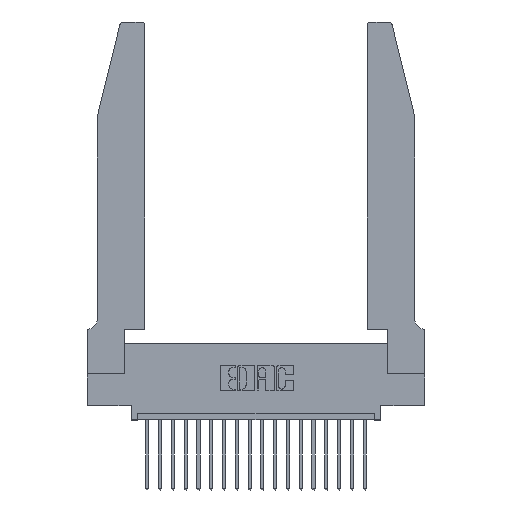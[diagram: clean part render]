
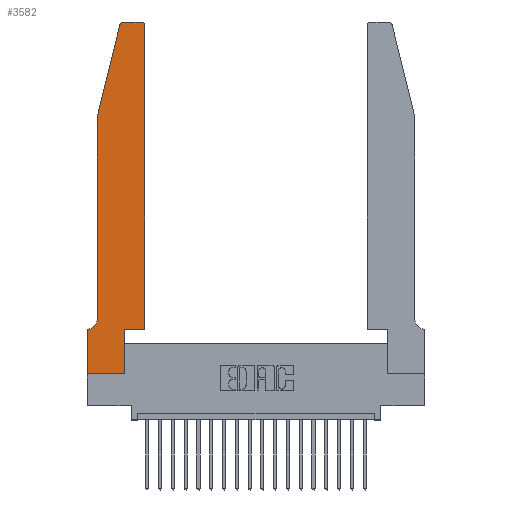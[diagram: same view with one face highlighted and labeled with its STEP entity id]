
A CAD part, top view. The second image highlights one B-rep face of the part: STEP entity #3582.
In plain terms, the highlighted planar face has unit normal (0, 0, 1).
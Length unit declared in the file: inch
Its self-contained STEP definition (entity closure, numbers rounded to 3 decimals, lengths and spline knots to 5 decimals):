
#22 = AXIS2_PLACEMENT_3D ( 'NONE', #5858, #7296, #2574 ) ;
#95 = CARTESIAN_POINT ( 'NONE',  ( 0.0755, 0.35, 0.37 ) ) ;
#312 = VERTEX_POINT ( 'NONE', #9934 ) ;
#774 = ORIENTED_EDGE ( 'NONE', *, *, #19800, .T. ) ;
#833 = ORIENTED_EDGE ( 'NONE', *, *, #8373, .T. ) ;
#1191 = CARTESIAN_POINT ( 'NONE',  ( 0.2865, 0., 0.37 ) ) ;
#1224 = DIRECTION ( 'NONE',  ( 0., 0., -1. ) ) ;
#1525 = VERTEX_POINT ( 'NONE', #7065 ) ;
#2114 = VERTEX_POINT ( 'NONE', #6592 ) ;
#2199 = DIRECTION ( 'NONE',  ( 1., 0., 0. ) ) ;
#2287 = CARTESIAN_POINT ( 'NONE',  ( 0.4505, 2.72, 0.37 ) ) ;
#2424 = CARTESIAN_POINT ( 'NONE',  ( 0.4505, 0.35, 0.37 ) ) ;
#2574 = DIRECTION ( 'NONE',  ( 1., 0., 0. ) ) ;
#2687 = CARTESIAN_POINT ( 'NONE',  ( 0., 0., 0.37 ) ) ;
#2689 = CARTESIAN_POINT ( 'NONE',  ( 0.4505, 0.35, 0.37 ) ) ;
#2951 = ORIENTED_EDGE ( 'NONE', *, *, #8413, .T. ) ;
#3290 = EDGE_CURVE ( 'NONE', #312, #1525, #5204, .T. ) ;
#3326 = CARTESIAN_POINT ( 'NONE',  ( 0.0755, 2., 0.37 ) ) ;
#3443 = DIRECTION ( 'NONE',  ( 0., 1., 0. ) ) ;
#3567 = VERTEX_POINT ( 'NONE', #18873 ) ;
#3582 = ADVANCED_FACE ( 'NONE', ( #17757 ), #12423, .T. ) ;
#4281 = CIRCLE ( 'NONE', #22, 0.03 ) ;
#4455 = EDGE_CURVE ( 'NONE', #10962, #15552, #10464, .T. ) ;
#4823 = VERTEX_POINT ( 'NONE', #2689 ) ;
#4848 = CIRCLE ( 'NONE', #10200, 0.07 ) ;
#5204 = LINE ( 'NONE', #95, #15141 ) ;
#5340 = DIRECTION ( 'NONE',  ( 1., 0., 0. ) ) ;
#5797 = ORIENTED_EDGE ( 'NONE', *, *, #17978, .T. ) ;
#5858 = CARTESIAN_POINT ( 'NONE',  ( 0.4205, 2.72, 0.37 ) ) ;
#5996 = VECTOR ( 'NONE', #9493, 39.37008 ) ;
#6002 = VERTEX_POINT ( 'NONE', #9565 ) ;
#6037 = VECTOR ( 'NONE', #3443, 39.37008 ) ;
#6434 = EDGE_CURVE ( 'NONE', #2114, #17561, #7002, .T. ) ;
#6592 = CARTESIAN_POINT ( 'NONE',  ( 0.25487, 2.72718, 0.37 ) ) ;
#6867 = DIRECTION ( 'NONE',  ( 1., 0., 0. ) ) ;
#7002 = LINE ( 'NONE', #3326, #19838 ) ;
#7065 = CARTESIAN_POINT ( 'NONE',  ( 0., 0.35, 0.37 ) ) ;
#7183 = ORIENTED_EDGE ( 'NONE', *, *, #11966, .T. ) ;
#7296 = DIRECTION ( 'NONE',  ( 0., 0., 1. ) ) ;
#7378 = ORIENTED_EDGE ( 'NONE', *, *, #11048, .T. ) ;
#7429 = EDGE_CURVE ( 'NONE', #9542, #10962, #13478, .T. ) ;
#8135 = CARTESIAN_POINT ( 'NONE',  ( 0.4205, 2.75, 0.37 ) ) ;
#8373 = EDGE_CURVE ( 'NONE', #1525, #9542, #9801, .T. ) ;
#8413 = EDGE_CURVE ( 'NONE', #3567, #312, #4848, .T. ) ;
#8762 = EDGE_LOOP ( 'NONE', ( #5797, #7378, #20561, #14508, #2951, #16219, #833, #11429, #17004, #13296, #774, #7183 ) ) ;
#9184 = VECTOR ( 'NONE', #9830, 39.37008 ) ;
#9236 = EDGE_CURVE ( 'NONE', #17561, #3567, #14203, .T. ) ;
#9493 = DIRECTION ( 'NONE',  ( 0., 1., 0. ) ) ;
#9542 = VERTEX_POINT ( 'NONE', #2687 ) ;
#9565 = CARTESIAN_POINT ( 'NONE',  ( 0.284, 2.75, 0.37 ) ) ;
#9631 = CARTESIAN_POINT ( 'NONE',  ( 0.0755, 2., 0.37 ) ) ;
#9801 = LINE ( 'NONE', #19722, #21322 ) ;
#9830 = DIRECTION ( 'NONE',  ( 1., 0., 0. ) ) ;
#9934 = CARTESIAN_POINT ( 'NONE',  ( 0.0055, 0.35, 0.37 ) ) ;
#10200 = AXIS2_PLACEMENT_3D ( 'NONE', #21321, #1224, #21167 ) ;
#10292 = DIRECTION ( 'NONE',  ( 0., -1., 0. ) ) ;
#10428 = LINE ( 'NONE', #12932, #5996 ) ;
#10464 = LINE ( 'NONE', #11978, #6037 ) ;
#10634 = AXIS2_PLACEMENT_3D ( 'NONE', #16898, #16827, #5340 ) ;
#10764 = CIRCLE ( 'NONE', #10634, 0.03 ) ;
#10874 = CARTESIAN_POINT ( 'NONE',  ( 0.2605, 2.75, 0.37 ) ) ;
#10962 = VERTEX_POINT ( 'NONE', #1191 ) ;
#11048 = EDGE_CURVE ( 'NONE', #6002, #2114, #10764, .T. ) ;
#11207 = EDGE_CURVE ( 'NONE', #15552, #4823, #18649, .T. ) ;
#11429 = ORIENTED_EDGE ( 'NONE', *, *, #7429, .T. ) ;
#11797 = DIRECTION ( 'NONE',  ( -1., 0., 0. ) ) ;
#11966 = EDGE_CURVE ( 'NONE', #13175, #20394, #4281, .T. ) ;
#11978 = CARTESIAN_POINT ( 'NONE',  ( 0.2865, 0.35, 0.37 ) ) ;
#12355 = CARTESIAN_POINT ( 'NONE',  ( 0., 0.35, 0.37 ) ) ;
#12423 = PLANE ( 'NONE',  #19418 ) ;
#12932 = CARTESIAN_POINT ( 'NONE',  ( 0.4505, 0.35, 0.37 ) ) ;
#13175 = VERTEX_POINT ( 'NONE', #2287 ) ;
#13296 = ORIENTED_EDGE ( 'NONE', *, *, #11207, .T. ) ;
#13346 = DIRECTION ( 'NONE',  ( -0.239, -0.971, 0. ) ) ;
#13478 = LINE ( 'NONE', #16605, #14808 ) ;
#13503 = LINE ( 'NONE', #10874, #16944 ) ;
#13936 = DIRECTION ( 'NONE',  ( 0., 0., 1. ) ) ;
#14203 = LINE ( 'NONE', #16958, #18138 ) ;
#14508 = ORIENTED_EDGE ( 'NONE', *, *, #9236, .T. ) ;
#14808 = VECTOR ( 'NONE', #6867, 39.37008 ) ;
#15141 = VECTOR ( 'NONE', #11797, 39.37008 ) ;
#15552 = VERTEX_POINT ( 'NONE', #20345 ) ;
#16219 = ORIENTED_EDGE ( 'NONE', *, *, #3290, .T. ) ;
#16268 = DIRECTION ( 'NONE',  ( 0., -1., 0. ) ) ;
#16605 = CARTESIAN_POINT ( 'NONE',  ( 0., 0., 0.37 ) ) ;
#16827 = DIRECTION ( 'NONE',  ( 0., 0., 1. ) ) ;
#16898 = CARTESIAN_POINT ( 'NONE',  ( 0.284, 2.72, 0.37 ) ) ;
#16944 = VECTOR ( 'NONE', #17397, 39.37008 ) ;
#16958 = CARTESIAN_POINT ( 'NONE',  ( 0.0755, 2., 0.37 ) ) ;
#17004 = ORIENTED_EDGE ( 'NONE', *, *, #4455, .T. ) ;
#17397 = DIRECTION ( 'NONE',  ( -1., 0., 0. ) ) ;
#17561 = VERTEX_POINT ( 'NONE', #9631 ) ;
#17757 = FACE_OUTER_BOUND ( 'NONE', #8762, .T. ) ;
#17978 = EDGE_CURVE ( 'NONE', #20394, #6002, #13503, .T. ) ;
#18138 = VECTOR ( 'NONE', #10292, 39.37008 ) ;
#18649 = LINE ( 'NONE', #2424, #9184 ) ;
#18873 = CARTESIAN_POINT ( 'NONE',  ( 0.0755, 0.42, 0.37 ) ) ;
#19418 = AXIS2_PLACEMENT_3D ( 'NONE', #12355, #13936, #2199 ) ;
#19722 = CARTESIAN_POINT ( 'NONE',  ( 0., 0., 0.37 ) ) ;
#19800 = EDGE_CURVE ( 'NONE', #4823, #13175, #10428, .T. ) ;
#19838 = VECTOR ( 'NONE', #13346, 39.37008 ) ;
#20345 = CARTESIAN_POINT ( 'NONE',  ( 0.2865, 0.35, 0.37 ) ) ;
#20394 = VERTEX_POINT ( 'NONE', #8135 ) ;
#20561 = ORIENTED_EDGE ( 'NONE', *, *, #6434, .T. ) ;
#21167 = DIRECTION ( 'NONE',  ( -1., 0., 0. ) ) ;
#21321 = CARTESIAN_POINT ( 'NONE',  ( 0.0055, 0.42, 0.37 ) ) ;
#21322 = VECTOR ( 'NONE', #16268, 39.37008 ) ;
